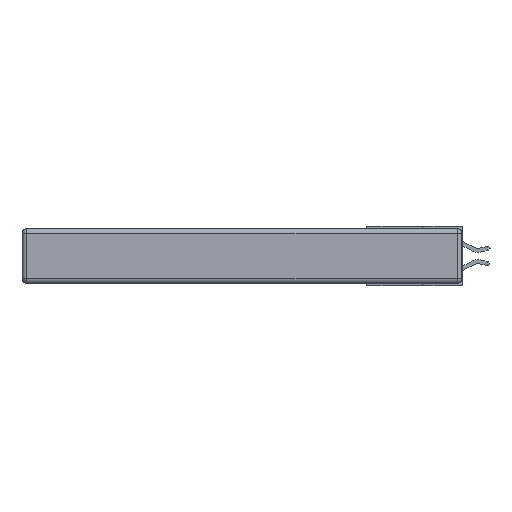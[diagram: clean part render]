
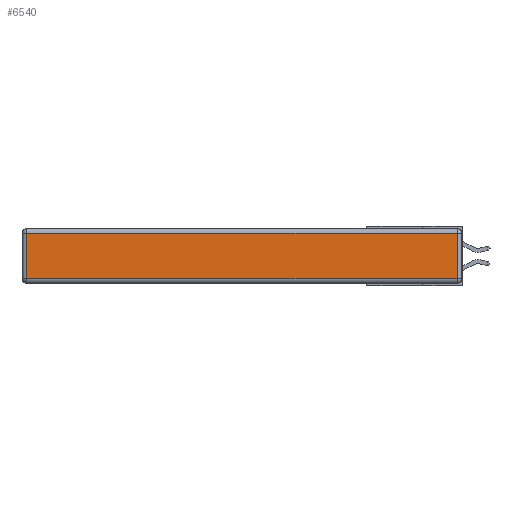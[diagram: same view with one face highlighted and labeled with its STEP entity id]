
A CAD part, left-side view. The second image highlights one B-rep face of the part: STEP entity #6540.
In plain terms, the highlighted planar face has unit normal (-1, 0, 0).
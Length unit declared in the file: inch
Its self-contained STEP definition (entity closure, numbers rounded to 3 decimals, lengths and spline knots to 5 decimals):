
#553 = CARTESIAN_POINT ( 'NONE',  ( 0., 2.72, -0.03 ) ) ;
#2447 = DIRECTION ( 'NONE',  ( 0., 0., -1. ) ) ;
#2475 = CARTESIAN_POINT ( 'NONE',  ( 0., 2.75, -0.03 ) ) ;
#4925 = CARTESIAN_POINT ( 'NONE',  ( 0., 0.03, -0.313 ) ) ;
#5290 = ORIENTED_EDGE ( 'NONE', *, *, #8110, .T. ) ;
#5658 = VECTOR ( 'NONE', #27703, 39.37008 ) ;
#5750 = DIRECTION ( 'NONE',  ( 0., 0., 1. ) ) ;
#5870 = CARTESIAN_POINT ( 'NONE',  ( 0., 0.03, -0.343 ) ) ;
#6540 = ADVANCED_FACE ( 'NONE', ( #20839 ), #10434, .T. ) ;
#7127 = AXIS2_PLACEMENT_3D ( 'NONE', #7920, #20336, #5750 ) ;
#7744 = CARTESIAN_POINT ( 'NONE',  ( 0., 0.03, -0.03 ) ) ;
#7920 = CARTESIAN_POINT ( 'NONE',  ( 0., 0., -0.343 ) ) ;
#8110 = EDGE_CURVE ( 'NONE', #27227, #25841, #24990, .T. ) ;
#9867 = CARTESIAN_POINT ( 'NONE',  ( 0., 2.72, -0.343 ) ) ;
#10434 = PLANE ( 'NONE',  #7127 ) ;
#10698 = CARTESIAN_POINT ( 'NONE',  ( 0., 0., -0.313 ) ) ;
#13574 = EDGE_LOOP ( 'NONE', ( #20703, #5290, #15223, #15955 ) ) ;
#14275 = VECTOR ( 'NONE', #2447, 39.37008 ) ;
#15223 = ORIENTED_EDGE ( 'NONE', *, *, #26838, .T. ) ;
#15955 = ORIENTED_EDGE ( 'NONE', *, *, #25366, .T. ) ;
#16100 = DIRECTION ( 'NONE',  ( 0., -1., 0. ) ) ;
#16490 = LINE ( 'NONE', #10698, #29016 ) ;
#17637 = VERTEX_POINT ( 'NONE', #553 ) ;
#20336 = DIRECTION ( 'NONE',  ( -1., 0., 0. ) ) ;
#20703 = ORIENTED_EDGE ( 'NONE', *, *, #27144, .T. ) ;
#20839 = FACE_OUTER_BOUND ( 'NONE', #13574, .T. ) ;
#20933 = CARTESIAN_POINT ( 'NONE',  ( 0., 2.72, -0.313 ) ) ;
#23538 = DIRECTION ( 'NONE',  ( 0., 0., 1. ) ) ;
#23818 = VERTEX_POINT ( 'NONE', #20933 ) ;
#24990 = LINE ( 'NONE', #5870, #31644 ) ;
#25366 = EDGE_CURVE ( 'NONE', #17637, #23818, #26751, .T. ) ;
#25528 = LINE ( 'NONE', #2475, #5658 ) ;
#25841 = VERTEX_POINT ( 'NONE', #7744 ) ;
#26751 = LINE ( 'NONE', #9867, #14275 ) ;
#26838 = EDGE_CURVE ( 'NONE', #25841, #17637, #25528, .T. ) ;
#27144 = EDGE_CURVE ( 'NONE', #23818, #27227, #16490, .T. ) ;
#27227 = VERTEX_POINT ( 'NONE', #4925 ) ;
#27703 = DIRECTION ( 'NONE',  ( 0., 1., 0. ) ) ;
#29016 = VECTOR ( 'NONE', #16100, 39.37008 ) ;
#31644 = VECTOR ( 'NONE', #23538, 39.37008 ) ;
